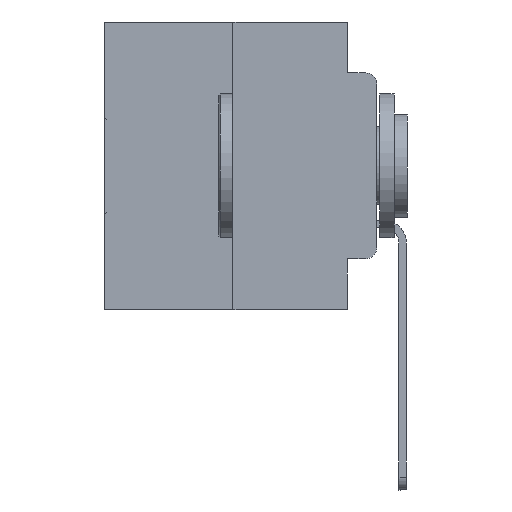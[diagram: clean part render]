
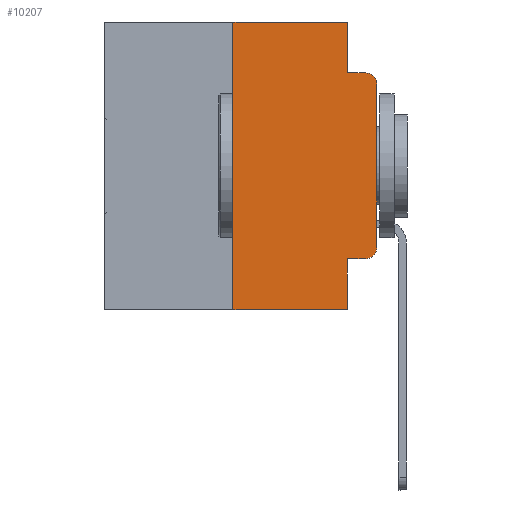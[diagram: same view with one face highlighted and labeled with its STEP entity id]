
A CAD part, left-side view. The second image highlights one B-rep face of the part: STEP entity #10207.
In plain terms, the highlighted planar face has unit normal (-1, 0, 0).
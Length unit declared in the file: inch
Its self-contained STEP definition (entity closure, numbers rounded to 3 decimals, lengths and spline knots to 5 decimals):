
#191 = CARTESIAN_POINT ( 'NONE',  ( 0., 0., 0. ) ) ;
#300 = EDGE_CURVE ( 'NONE', #29544, #10781, #25913, .T. ) ;
#480 = VECTOR ( 'NONE', #28296, 39.37008 ) ;
#832 = CARTESIAN_POINT ( 'NONE',  ( 0., 0., -0.3915 ) ) ;
#1495 = DIRECTION ( 'NONE',  ( 0., -1., 0. ) ) ;
#1528 = CARTESIAN_POINT ( 'NONE',  ( 0., 0.25, 0. ) ) ;
#1564 = VERTEX_POINT ( 'NONE', #3950 ) ;
#2078 = EDGE_CURVE ( 'NONE', #16568, #8950, #2732, .T. ) ;
#2135 = EDGE_LOOP ( 'NONE', ( #5345, #26853, #17339, #25080, #7262, #12314, #7630, #15900, #28335, #10182 ) ) ;
#2236 = LINE ( 'NONE', #18977, #26476 ) ;
#2727 = CIRCLE ( 'NONE', #11202, 0.02 ) ;
#2732 = LINE ( 'NONE', #1528, #21458 ) ;
#3003 = CARTESIAN_POINT ( 'NONE',  ( 0., 0.25, 0. ) ) ;
#3466 = PLANE ( 'NONE',  #14060 ) ;
#3744 = EDGE_CURVE ( 'NONE', #11978, #1564, #2236, .T. ) ;
#3950 = CARTESIAN_POINT ( 'NONE',  ( 0., 0.051, -0.0885 ) ) ;
#5237 = VECTOR ( 'NONE', #1495, 39.37008 ) ;
#5345 = ORIENTED_EDGE ( 'NONE', *, *, #10136, .T. ) ;
#5817 = VERTEX_POINT ( 'NONE', #832 ) ;
#7023 = EDGE_CURVE ( 'NONE', #1564, #14768, #18595, .T. ) ;
#7262 = ORIENTED_EDGE ( 'NONE', *, *, #13451, .F. ) ;
#7630 = ORIENTED_EDGE ( 'NONE', *, *, #22993, .T. ) ;
#8209 = AXIS2_PLACEMENT_3D ( 'NONE', #11122, #27369, #13462 ) ;
#8304 = CARTESIAN_POINT ( 'NONE',  ( 0., 0.473, 0. ) ) ;
#8571 = EDGE_CURVE ( 'NONE', #27481, #14768, #13174, .T. ) ;
#8950 = VERTEX_POINT ( 'NONE', #3003 ) ;
#9000 = CARTESIAN_POINT ( 'NONE',  ( 0., 0.051, 0. ) ) ;
#9877 = CARTESIAN_POINT ( 'NONE',  ( 0., 0., -0.1085 ) ) ;
#10136 = EDGE_CURVE ( 'NONE', #5817, #27481, #25118, .T. ) ;
#10182 = ORIENTED_EDGE ( 'NONE', *, *, #26285, .T. ) ;
#10207 = ADVANCED_FACE ( 'NONE', ( #16655 ), #3466, .F. ) ;
#10626 = DIRECTION ( 'NONE',  ( 0., 0., -1. ) ) ;
#10781 = VERTEX_POINT ( 'NONE', #14926 ) ;
#10888 = DIRECTION ( 'NONE',  ( 0., 0., 1. ) ) ;
#11122 = CARTESIAN_POINT ( 'NONE',  ( 0., 0.02, -0.1085 ) ) ;
#11202 = AXIS2_PLACEMENT_3D ( 'NONE', #11801, #28055, #14123 ) ;
#11686 = CARTESIAN_POINT ( 'NONE',  ( 0., 0.473, -0.5 ) ) ;
#11711 = VECTOR ( 'NONE', #28976, 39.37008 ) ;
#11801 = CARTESIAN_POINT ( 'NONE',  ( 0., 0.02, -0.3915 ) ) ;
#11978 = VERTEX_POINT ( 'NONE', #9000 ) ;
#11982 = VECTOR ( 'NONE', #21588, 39.37008 ) ;
#12314 = ORIENTED_EDGE ( 'NONE', *, *, #2078, .F. ) ;
#13174 = CIRCLE ( 'NONE', #8209, 0.02 ) ;
#13451 = EDGE_CURVE ( 'NONE', #8950, #11978, #20187, .T. ) ;
#13462 = DIRECTION ( 'NONE',  ( 0., 0., -1. ) ) ;
#14017 = DIRECTION ( 'NONE',  ( 0., -1., 0. ) ) ;
#14060 = AXIS2_PLACEMENT_3D ( 'NONE', #8304, #24580, #10626 ) ;
#14123 = DIRECTION ( 'NONE',  ( 0., 0., -1. ) ) ;
#14390 = DIRECTION ( 'NONE',  ( 0., 0., -1. ) ) ;
#14687 = LINE ( 'NONE', #11686, #20172 ) ;
#14768 = VERTEX_POINT ( 'NONE', #20964 ) ;
#14926 = CARTESIAN_POINT ( 'NONE',  ( 0., 0.051, -0.5 ) ) ;
#15900 = ORIENTED_EDGE ( 'NONE', *, *, #300, .F. ) ;
#16337 = CARTESIAN_POINT ( 'NONE',  ( 0., 0.25, -0.5 ) ) ;
#16520 = CARTESIAN_POINT ( 'NONE',  ( 0., 0.051, -0.4115 ) ) ;
#16568 = VERTEX_POINT ( 'NONE', #16337 ) ;
#16655 = FACE_OUTER_BOUND ( 'NONE', #2135, .T. ) ;
#17258 = CARTESIAN_POINT ( 'NONE',  ( 0., 0.051, -0.0885 ) ) ;
#17339 = ORIENTED_EDGE ( 'NONE', *, *, #7023, .F. ) ;
#18595 = LINE ( 'NONE', #17258, #11711 ) ;
#18693 = VERTEX_POINT ( 'NONE', #20039 ) ;
#18977 = CARTESIAN_POINT ( 'NONE',  ( 0., 0.051, 0. ) ) ;
#20039 = CARTESIAN_POINT ( 'NONE',  ( 0., 0.02, -0.4115 ) ) ;
#20172 = VECTOR ( 'NONE', #14017, 39.37008 ) ;
#20187 = LINE ( 'NONE', #28198, #480 ) ;
#20964 = CARTESIAN_POINT ( 'NONE',  ( 0., 0.02, -0.0885 ) ) ;
#21458 = VECTOR ( 'NONE', #10888, 39.37008 ) ;
#21588 = DIRECTION ( 'NONE',  ( 0., 0., 1. ) ) ;
#22993 = EDGE_CURVE ( 'NONE', #16568, #10781, #14687, .T. ) ;
#24580 = DIRECTION ( 'NONE',  ( 1., 0., 0. ) ) ;
#25010 = CARTESIAN_POINT ( 'NONE',  ( 0., 0.051, -0.4115 ) ) ;
#25080 = ORIENTED_EDGE ( 'NONE', *, *, #3744, .F. ) ;
#25118 = LINE ( 'NONE', #191, #11982 ) ;
#25201 = VECTOR ( 'NONE', #28415, 39.37008 ) ;
#25913 = LINE ( 'NONE', #29918, #25201 ) ;
#26285 = EDGE_CURVE ( 'NONE', #18693, #5817, #2727, .T. ) ;
#26476 = VECTOR ( 'NONE', #14390, 39.37008 ) ;
#26853 = ORIENTED_EDGE ( 'NONE', *, *, #8571, .T. ) ;
#27369 = DIRECTION ( 'NONE',  ( -1., 0., 0. ) ) ;
#27481 = VERTEX_POINT ( 'NONE', #9877 ) ;
#27826 = EDGE_CURVE ( 'NONE', #29544, #18693, #29925, .T. ) ;
#28055 = DIRECTION ( 'NONE',  ( -1., 0., 0. ) ) ;
#28198 = CARTESIAN_POINT ( 'NONE',  ( 0., 0.473, 0. ) ) ;
#28296 = DIRECTION ( 'NONE',  ( 0., -1., 0. ) ) ;
#28335 = ORIENTED_EDGE ( 'NONE', *, *, #27826, .T. ) ;
#28415 = DIRECTION ( 'NONE',  ( 0., 0., -1. ) ) ;
#28976 = DIRECTION ( 'NONE',  ( 0., -1., 0. ) ) ;
#29544 = VERTEX_POINT ( 'NONE', #16520 ) ;
#29918 = CARTESIAN_POINT ( 'NONE',  ( 0., 0.051, 0. ) ) ;
#29925 = LINE ( 'NONE', #25010, #5237 ) ;
